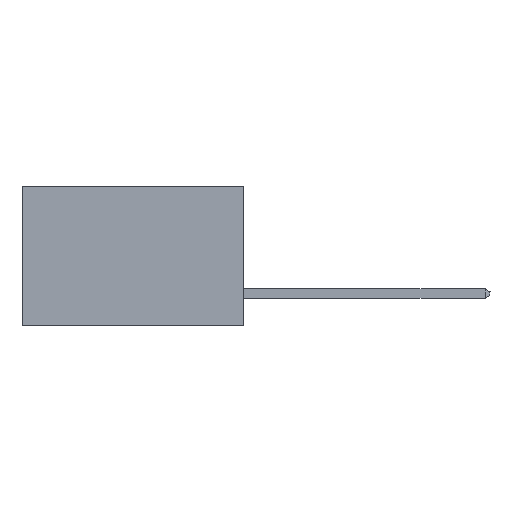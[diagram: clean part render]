
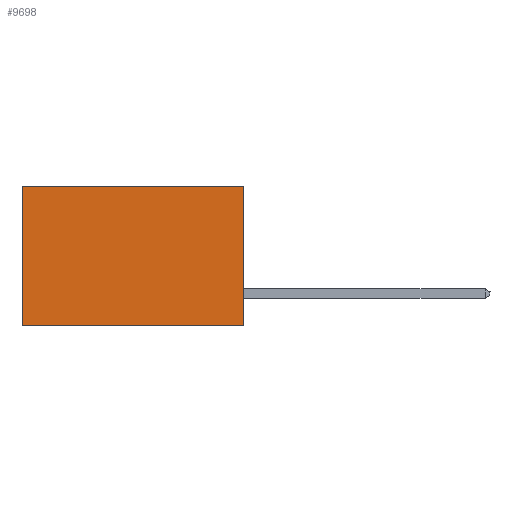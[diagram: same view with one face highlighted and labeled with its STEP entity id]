
A CAD part, left-side view. The second image highlights one B-rep face of the part: STEP entity #9698.
In plain terms, the highlighted planar face has unit normal (-1, 0, 0).
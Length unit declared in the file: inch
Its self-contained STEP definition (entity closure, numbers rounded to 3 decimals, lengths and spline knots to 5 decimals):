
#570 = VERTEX_POINT ( 'NONE', #16487 ) ;
#861 = VECTOR ( 'NONE', #4216, 39.37008 ) ;
#1343 = EDGE_CURVE ( 'NONE', #570, #9192, #5394, .T. ) ;
#1408 = CARTESIAN_POINT ( 'NONE',  ( 0.277, 0., 0. ) ) ;
#1727 = ORIENTED_EDGE ( 'NONE', *, *, #3711, .F. ) ;
#2648 = DIRECTION ( 'NONE',  ( 1., 0., 0. ) ) ;
#3316 = CARTESIAN_POINT ( 'NONE',  ( 0.277, 0., -0.37 ) ) ;
#3653 = EDGE_CURVE ( 'NONE', #5810, #10183, #8094, .T. ) ;
#3711 = EDGE_CURVE ( 'NONE', #570, #5810, #10185, .T. ) ;
#4216 = DIRECTION ( 'NONE',  ( 0., 1., 0. ) ) ;
#4892 = CARTESIAN_POINT ( 'NONE',  ( 0.277, 0., -0.37 ) ) ;
#4958 = VECTOR ( 'NONE', #14739, 39.37008 ) ;
#5394 = LINE ( 'NONE', #1408, #4958 ) ;
#5810 = VERTEX_POINT ( 'NONE', #3316 ) ;
#6722 = PLANE ( 'NONE',  #7645 ) ;
#7412 = CARTESIAN_POINT ( 'NONE',  ( 0.277, 0.59, -0.37 ) ) ;
#7645 = AXIS2_PLACEMENT_3D ( 'NONE', #10502, #2648, #11725 ) ;
#8094 = LINE ( 'NONE', #4892, #861 ) ;
#8505 = ORIENTED_EDGE ( 'NONE', *, *, #8687, .T. ) ;
#8687 = EDGE_CURVE ( 'NONE', #9192, #10183, #15890, .T. ) ;
#9192 = VERTEX_POINT ( 'NONE', #12323 ) ;
#9552 = EDGE_LOOP ( 'NONE', ( #8505, #14967, #1727, #12495 ) ) ;
#9698 = ADVANCED_FACE ( 'NONE', ( #14391 ), #6722, .F. ) ;
#10183 = VERTEX_POINT ( 'NONE', #7412 ) ;
#10185 = LINE ( 'NONE', #15374, #16267 ) ;
#10502 = CARTESIAN_POINT ( 'NONE',  ( 0.277, 0., -0.37 ) ) ;
#11725 = DIRECTION ( 'NONE',  ( 0., 0., -1. ) ) ;
#12323 = CARTESIAN_POINT ( 'NONE',  ( 0.277, 0.59, 0. ) ) ;
#12495 = ORIENTED_EDGE ( 'NONE', *, *, #1343, .T. ) ;
#14391 = FACE_OUTER_BOUND ( 'NONE', #9552, .T. ) ;
#14739 = DIRECTION ( 'NONE',  ( 0., 1., 0. ) ) ;
#14967 = ORIENTED_EDGE ( 'NONE', *, *, #3653, .F. ) ;
#15100 = CARTESIAN_POINT ( 'NONE',  ( 0.277, 0.59, -0.37 ) ) ;
#15374 = CARTESIAN_POINT ( 'NONE',  ( 0.277, 0., -0.37 ) ) ;
#15890 = LINE ( 'NONE', #15100, #16261 ) ;
#16231 = DIRECTION ( 'NONE',  ( 0., 0., -1. ) ) ;
#16261 = VECTOR ( 'NONE', #16306, 39.37008 ) ;
#16267 = VECTOR ( 'NONE', #16231, 39.37008 ) ;
#16306 = DIRECTION ( 'NONE',  ( 0., 0., -1. ) ) ;
#16487 = CARTESIAN_POINT ( 'NONE',  ( 0.277, 0., 0. ) ) ;
